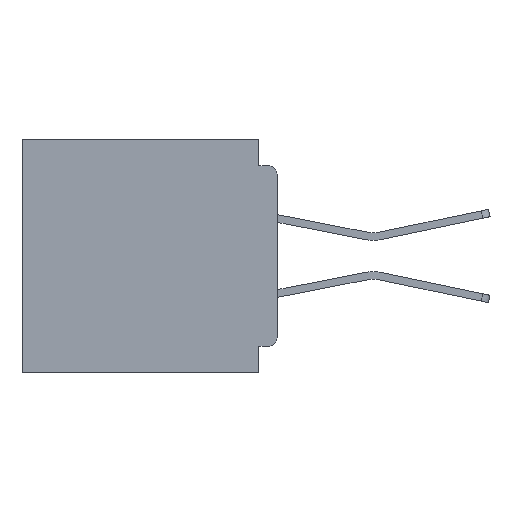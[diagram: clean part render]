
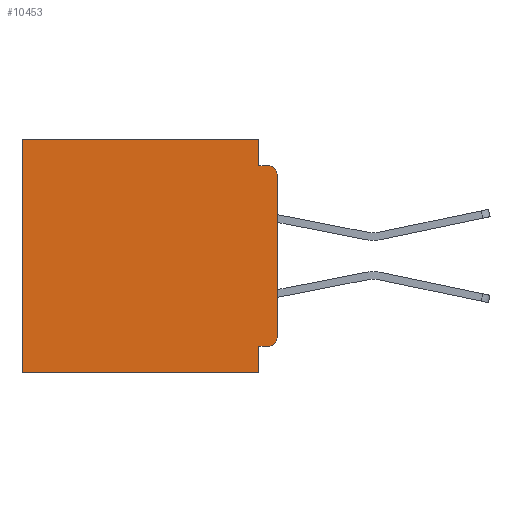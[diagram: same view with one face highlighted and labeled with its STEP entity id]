
A CAD part, left-side view. The second image highlights one B-rep face of the part: STEP entity #10453.
In plain terms, the highlighted planar face has unit normal (-1, 0, 0).
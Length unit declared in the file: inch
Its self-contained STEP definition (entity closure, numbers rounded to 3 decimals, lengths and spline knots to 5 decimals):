
#24 = DIRECTION ( 'NONE',  ( 0., 0., -1. ) ) ;
#740 = VECTOR ( 'NONE', #54345, 39.37008 ) ;
#1744 = ORIENTED_EDGE ( 'NONE', *, *, #20139, .F. ) ;
#3077 = EDGE_LOOP ( 'NONE', ( #47812, #5661, #13506, #55488, #38998, #13843, #10791, #1744, #27774, #57063 ) ) ;
#3472 = LINE ( 'NONE', #60357, #26834 ) ;
#3967 = DIRECTION ( 'NONE',  ( 0., 1., 0. ) ) ;
#4545 = DIRECTION ( 'NONE',  ( 0., -1., 0. ) ) ;
#4973 = CARTESIAN_POINT ( 'NONE',  ( 0.3, 0.015, -0.06 ) ) ;
#5305 = DIRECTION ( 'NONE',  ( 0., 0., -1. ) ) ;
#5383 = DIRECTION ( 'NONE',  ( 0., 0., -1. ) ) ;
#5661 = ORIENTED_EDGE ( 'NONE', *, *, #30994, .T. ) ;
#7232 = VERTEX_POINT ( 'NONE', #44435 ) ;
#7583 = CARTESIAN_POINT ( 'NONE',  ( 0.3, 0., -0.34 ) ) ;
#8034 = EDGE_CURVE ( 'NONE', #7232, #18590, #33052, .T. ) ;
#8054 = VECTOR ( 'NONE', #41783, 39.37008 ) ;
#9693 = DIRECTION ( 'NONE',  ( 0., 0., -1. ) ) ;
#10453 = ADVANCED_FACE ( 'NONE', ( #47352 ), #52576, .F. ) ;
#10791 = ORIENTED_EDGE ( 'NONE', *, *, #8034, .F. ) ;
#11739 = CARTESIAN_POINT ( 'NONE',  ( 0.3, 0.031, -0.355 ) ) ;
#11884 = AXIS2_PLACEMENT_3D ( 'NONE', #55852, #27973, #24 ) ;
#13273 = VECTOR ( 'NONE', #42780, 39.37008 ) ;
#13395 = CARTESIAN_POINT ( 'NONE',  ( 0.3, 0., -0.4 ) ) ;
#13506 = ORIENTED_EDGE ( 'NONE', *, *, #31409, .F. ) ;
#13843 = ORIENTED_EDGE ( 'NONE', *, *, #40921, .T. ) ;
#14658 = LINE ( 'NONE', #35590, #50322 ) ;
#16143 = CARTESIAN_POINT ( 'NONE',  ( 0.3, 0.031, 0. ) ) ;
#17178 = VECTOR ( 'NONE', #5383, 39.37008 ) ;
#18434 = CARTESIAN_POINT ( 'NONE',  ( 0.3, 0.015, -0.045 ) ) ;
#18459 = EDGE_CURVE ( 'NONE', #44379, #55856, #21428, .T. ) ;
#18590 = VERTEX_POINT ( 'NONE', #42818 ) ;
#19392 = CARTESIAN_POINT ( 'NONE',  ( 0.3, 0.437, -0.4 ) ) ;
#19737 = CARTESIAN_POINT ( 'NONE',  ( 0.3, 0.437, 0. ) ) ;
#20037 = EDGE_CURVE ( 'NONE', #38448, #55856, #45248, .T. ) ;
#20139 = EDGE_CURVE ( 'NONE', #38279, #7232, #25572, .T. ) ;
#21428 = CIRCLE ( 'NONE', #11884, 0.015 ) ;
#22118 = VERTEX_POINT ( 'NONE', #16143 ) ;
#22173 = CARTESIAN_POINT ( 'NONE',  ( 0.3, 0.015, -0.355 ) ) ;
#24065 = EDGE_CURVE ( 'NONE', #22118, #53149, #14658, .T. ) ;
#24069 = EDGE_CURVE ( 'NONE', #44379, #38279, #37951, .T. ) ;
#24133 = VECTOR ( 'NONE', #5305, 39.37008 ) ;
#24705 = DIRECTION ( 'NONE',  ( 1., 0., 0. ) ) ;
#25572 = LINE ( 'NONE', #47089, #24133 ) ;
#26834 = VECTOR ( 'NONE', #4545, 39.37008 ) ;
#26988 = EDGE_CURVE ( 'NONE', #22118, #56533, #30990, .T. ) ;
#27099 = LINE ( 'NONE', #19392, #13273 ) ;
#27774 = ORIENTED_EDGE ( 'NONE', *, *, #24069, .F. ) ;
#27973 = DIRECTION ( 'NONE',  ( -1., 0., 0. ) ) ;
#30990 = LINE ( 'NONE', #37985, #17178 ) ;
#30994 = EDGE_CURVE ( 'NONE', #38448, #47280, #39316, .T. ) ;
#31135 = CARTESIAN_POINT ( 'NONE',  ( 0.3, 0.031, -0.045 ) ) ;
#31409 = EDGE_CURVE ( 'NONE', #56533, #47280, #3472, .T. ) ;
#33052 = LINE ( 'NONE', #13395, #54911 ) ;
#35590 = CARTESIAN_POINT ( 'NONE',  ( 0.3, 0., 0. ) ) ;
#36126 = CARTESIAN_POINT ( 'NONE',  ( 0.3, 0., -0.06 ) ) ;
#37089 = CARTESIAN_POINT ( 'NONE',  ( 0.3, 0., -0.4 ) ) ;
#37586 = DIRECTION ( 'NONE',  ( -1., 0., 0. ) ) ;
#37951 = LINE ( 'NONE', #49637, #740 ) ;
#37985 = CARTESIAN_POINT ( 'NONE',  ( 0.3, 0.031, 0. ) ) ;
#38279 = VERTEX_POINT ( 'NONE', #11739 ) ;
#38448 = VERTEX_POINT ( 'NONE', #36126 ) ;
#38537 = CARTESIAN_POINT ( 'NONE',  ( 0.3, 0., -0.4 ) ) ;
#38998 = ORIENTED_EDGE ( 'NONE', *, *, #24065, .T. ) ;
#39316 = CIRCLE ( 'NONE', #51398, 0.015 ) ;
#40301 = DIRECTION ( 'NONE',  ( 0., 1., 0. ) ) ;
#40921 = EDGE_CURVE ( 'NONE', #53149, #18590, #27099, .T. ) ;
#41783 = DIRECTION ( 'NONE',  ( 0., 0., -1. ) ) ;
#42780 = DIRECTION ( 'NONE',  ( 0., 0., -1. ) ) ;
#42818 = CARTESIAN_POINT ( 'NONE',  ( 0.3, 0.437, -0.4 ) ) ;
#44379 = VERTEX_POINT ( 'NONE', #22173 ) ;
#44435 = CARTESIAN_POINT ( 'NONE',  ( 0.3, 0.031, -0.4 ) ) ;
#45248 = LINE ( 'NONE', #37089, #8054 ) ;
#46183 = AXIS2_PLACEMENT_3D ( 'NONE', #38537, #24705, #57248 ) ;
#47089 = CARTESIAN_POINT ( 'NONE',  ( 0.3, 0.031, -0.4 ) ) ;
#47280 = VERTEX_POINT ( 'NONE', #18434 ) ;
#47352 = FACE_OUTER_BOUND ( 'NONE', #3077, .T. ) ;
#47812 = ORIENTED_EDGE ( 'NONE', *, *, #20037, .F. ) ;
#49637 = CARTESIAN_POINT ( 'NONE',  ( 0.3, 0., -0.355 ) ) ;
#50322 = VECTOR ( 'NONE', #40301, 39.37008 ) ;
#51398 = AXIS2_PLACEMENT_3D ( 'NONE', #4973, #37586, #9693 ) ;
#52576 = PLANE ( 'NONE',  #46183 ) ;
#53149 = VERTEX_POINT ( 'NONE', #19737 ) ;
#54345 = DIRECTION ( 'NONE',  ( 0., 1., 0. ) ) ;
#54911 = VECTOR ( 'NONE', #3967, 39.37008 ) ;
#55488 = ORIENTED_EDGE ( 'NONE', *, *, #26988, .F. ) ;
#55852 = CARTESIAN_POINT ( 'NONE',  ( 0.3, 0.015, -0.34 ) ) ;
#55856 = VERTEX_POINT ( 'NONE', #7583 ) ;
#56533 = VERTEX_POINT ( 'NONE', #31135 ) ;
#57063 = ORIENTED_EDGE ( 'NONE', *, *, #18459, .T. ) ;
#57248 = DIRECTION ( 'NONE',  ( 0., 0., -1. ) ) ;
#60357 = CARTESIAN_POINT ( 'NONE',  ( 0.3, 0., -0.045 ) ) ;
